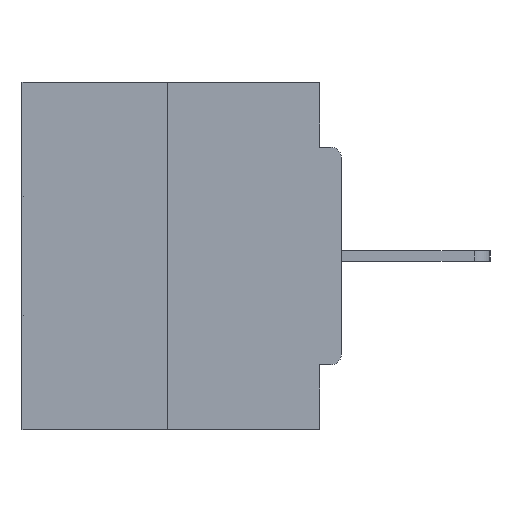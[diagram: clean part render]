
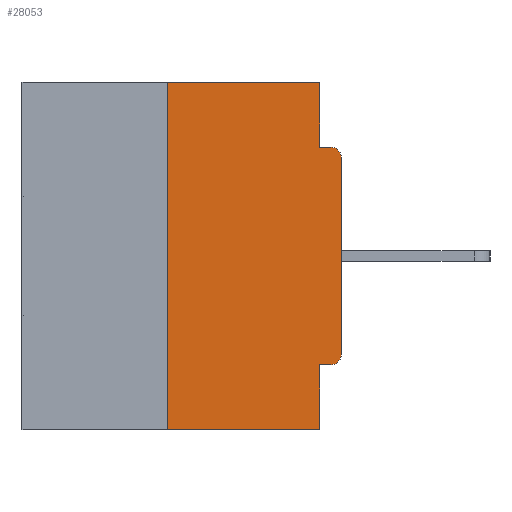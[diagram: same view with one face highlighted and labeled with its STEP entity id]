
A CAD part, left-side view. The second image highlights one B-rep face of the part: STEP entity #28053.
In plain terms, the highlighted planar face has unit normal (-1, 0, 0).
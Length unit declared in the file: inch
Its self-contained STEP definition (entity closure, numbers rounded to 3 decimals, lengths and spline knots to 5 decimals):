
#746 = CIRCLE ( 'NONE', #23728, 0.015 ) ;
#1286 = CARTESIAN_POINT ( 'NONE',  ( 0., 0.25, 0. ) ) ;
#1557 = LINE ( 'NONE', #30210, #17764 ) ;
#1722 = DIRECTION ( 'NONE',  ( 0., 1., 0. ) ) ;
#2313 = VERTEX_POINT ( 'NONE', #30278 ) ;
#2361 = VERTEX_POINT ( 'NONE', #27540 ) ;
#2517 = CARTESIAN_POINT ( 'NONE',  ( 0., 0.031, -0.4065 ) ) ;
#2560 = LINE ( 'NONE', #13037, #33591 ) ;
#2795 = DIRECTION ( 'NONE',  ( 0., 0., -1. ) ) ;
#2883 = CARTESIAN_POINT ( 'NONE',  ( 0., 0.46, 0. ) ) ;
#3086 = VERTEX_POINT ( 'NONE', #16144 ) ;
#3881 = LINE ( 'NONE', #1286, #20936 ) ;
#4020 = CARTESIAN_POINT ( 'NONE',  ( 0., 0., -0.0935 ) ) ;
#5741 = LINE ( 'NONE', #10891, #9352 ) ;
#6282 = DIRECTION ( 'NONE',  ( 0., 0., 1. ) ) ;
#6346 = VECTOR ( 'NONE', #31218, 39.37008 ) ;
#6592 = VERTEX_POINT ( 'NONE', #2517 ) ;
#6761 = LINE ( 'NONE', #4020, #16183 ) ;
#7013 = EDGE_CURVE ( 'NONE', #25040, #13477, #5741, .T. ) ;
#7123 = CARTESIAN_POINT ( 'NONE',  ( 0., 0.031, -0.5 ) ) ;
#7162 = ORIENTED_EDGE ( 'NONE', *, *, #21918, .T. ) ;
#7623 = CARTESIAN_POINT ( 'NONE',  ( 0., 0.25, 0. ) ) ;
#8002 = VERTEX_POINT ( 'NONE', #8872 ) ;
#8140 = EDGE_CURVE ( 'NONE', #2313, #15522, #30454, .T. ) ;
#8457 = CARTESIAN_POINT ( 'NONE',  ( 0., 0.015, -0.1085 ) ) ;
#8571 = DIRECTION ( 'NONE',  ( 0., 0., -1. ) ) ;
#8872 = CARTESIAN_POINT ( 'NONE',  ( 0., 0.015, -0.0935 ) ) ;
#9206 = CARTESIAN_POINT ( 'NONE',  ( 0., 0., 0. ) ) ;
#9352 = VECTOR ( 'NONE', #13643, 39.37008 ) ;
#9773 = LINE ( 'NONE', #14749, #26253 ) ;
#10655 = EDGE_CURVE ( 'NONE', #3086, #8002, #6761, .T. ) ;
#10891 = CARTESIAN_POINT ( 'NONE',  ( 0., 0.46, -0.5 ) ) ;
#12476 = CARTESIAN_POINT ( 'NONE',  ( 0., 0.015, -0.3915 ) ) ;
#13037 = CARTESIAN_POINT ( 'NONE',  ( 0., 0.031, 0. ) ) ;
#13365 = CARTESIAN_POINT ( 'NONE',  ( 0., 0.031, -0.5 ) ) ;
#13477 = VERTEX_POINT ( 'NONE', #7123 ) ;
#13607 = CARTESIAN_POINT ( 'NONE',  ( 0., 0.031, 0. ) ) ;
#13643 = DIRECTION ( 'NONE',  ( 0., -1., 0. ) ) ;
#13863 = DIRECTION ( 'NONE',  ( 0., 0., -1. ) ) ;
#14685 = DIRECTION ( 'NONE',  ( 0., 0., 1. ) ) ;
#14749 = CARTESIAN_POINT ( 'NONE',  ( 0., 0.46, 0. ) ) ;
#15036 = DIRECTION ( 'NONE',  ( 0., 0., -1. ) ) ;
#15091 = CARTESIAN_POINT ( 'NONE',  ( 0., 0.25, -0.5 ) ) ;
#15143 = DIRECTION ( 'NONE',  ( 0., -1., 0. ) ) ;
#15522 = VERTEX_POINT ( 'NONE', #17999 ) ;
#15859 = EDGE_LOOP ( 'NONE', ( #20991, #27377, #30134, #21199, #16070, #7162, #18299, #20298, #28608, #29090 ) ) ;
#15924 = PLANE ( 'NONE',  #22550 ) ;
#16070 = ORIENTED_EDGE ( 'NONE', *, *, #24809, .F. ) ;
#16144 = CARTESIAN_POINT ( 'NONE',  ( 0., 0.031, -0.0935 ) ) ;
#16183 = VECTOR ( 'NONE', #15143, 39.37008 ) ;
#17539 = EDGE_CURVE ( 'NONE', #15522, #8002, #19061, .T. ) ;
#17764 = VECTOR ( 'NONE', #1722, 39.37008 ) ;
#17999 = CARTESIAN_POINT ( 'NONE',  ( 0., 0., -0.1085 ) ) ;
#18299 = ORIENTED_EDGE ( 'NONE', *, *, #8140, .T. ) ;
#18665 = DIRECTION ( 'NONE',  ( 1., 0., 0. ) ) ;
#19061 = CIRCLE ( 'NONE', #31133, 0.015 ) ;
#20258 = EDGE_CURVE ( 'NONE', #29360, #25955, #9773, .T. ) ;
#20298 = ORIENTED_EDGE ( 'NONE', *, *, #17539, .T. ) ;
#20936 = VECTOR ( 'NONE', #6282, 39.37008 ) ;
#20982 = EDGE_CURVE ( 'NONE', #25040, #29360, #3881, .T. ) ;
#20991 = ORIENTED_EDGE ( 'NONE', *, *, #20258, .F. ) ;
#21199 = ORIENTED_EDGE ( 'NONE', *, *, #31416, .F. ) ;
#21918 = EDGE_CURVE ( 'NONE', #2361, #2313, #746, .T. ) ;
#22458 = DIRECTION ( 'NONE',  ( 0., -1., 0. ) ) ;
#22550 = AXIS2_PLACEMENT_3D ( 'NONE', #2883, #18665, #13863 ) ;
#23447 = EDGE_CURVE ( 'NONE', #25955, #3086, #2560, .T. ) ;
#23728 = AXIS2_PLACEMENT_3D ( 'NONE', #12476, #25495, #15036 ) ;
#24809 = EDGE_CURVE ( 'NONE', #2361, #6592, #1557, .T. ) ;
#25040 = VERTEX_POINT ( 'NONE', #15091 ) ;
#25495 = DIRECTION ( 'NONE',  ( -1., 0., 0. ) ) ;
#25955 = VERTEX_POINT ( 'NONE', #13607 ) ;
#26253 = VECTOR ( 'NONE', #22458, 39.37008 ) ;
#26392 = FACE_OUTER_BOUND ( 'NONE', #15859, .T. ) ;
#27377 = ORIENTED_EDGE ( 'NONE', *, *, #20982, .F. ) ;
#27540 = CARTESIAN_POINT ( 'NONE',  ( 0., 0.015, -0.4065 ) ) ;
#28053 = ADVANCED_FACE ( 'NONE', ( #26392 ), #15924, .F. ) ;
#28608 = ORIENTED_EDGE ( 'NONE', *, *, #10655, .F. ) ;
#28789 = LINE ( 'NONE', #13365, #6346 ) ;
#29090 = ORIENTED_EDGE ( 'NONE', *, *, #23447, .F. ) ;
#29360 = VERTEX_POINT ( 'NONE', #7623 ) ;
#29374 = DIRECTION ( 'NONE',  ( -1., 0., 0. ) ) ;
#30134 = ORIENTED_EDGE ( 'NONE', *, *, #7013, .T. ) ;
#30210 = CARTESIAN_POINT ( 'NONE',  ( 0., 0., -0.4065 ) ) ;
#30278 = CARTESIAN_POINT ( 'NONE',  ( 0., 0., -0.3915 ) ) ;
#30454 = LINE ( 'NONE', #9206, #31859 ) ;
#31133 = AXIS2_PLACEMENT_3D ( 'NONE', #8457, #29374, #2795 ) ;
#31218 = DIRECTION ( 'NONE',  ( 0., 0., -1. ) ) ;
#31416 = EDGE_CURVE ( 'NONE', #6592, #13477, #28789, .T. ) ;
#31859 = VECTOR ( 'NONE', #14685, 39.37008 ) ;
#33591 = VECTOR ( 'NONE', #8571, 39.37008 ) ;
